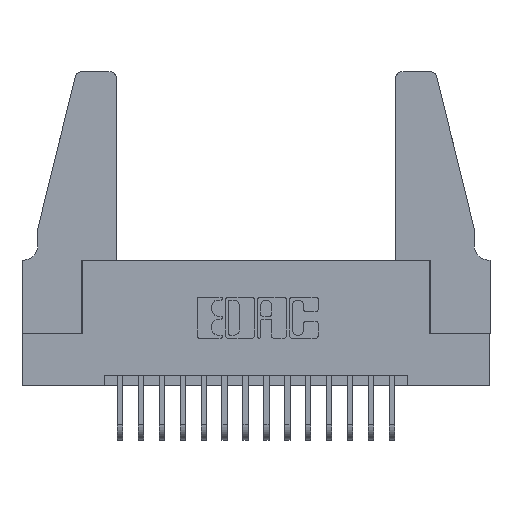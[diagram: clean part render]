
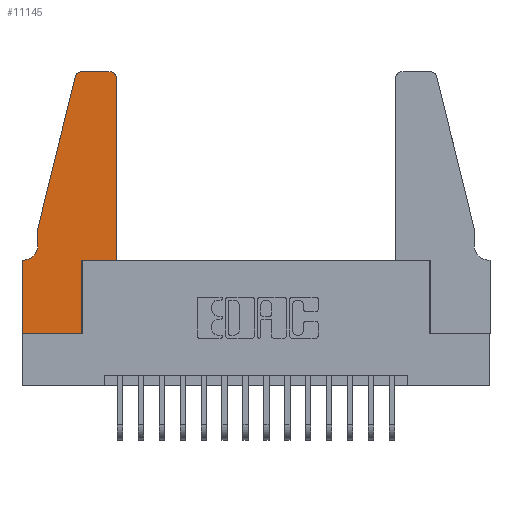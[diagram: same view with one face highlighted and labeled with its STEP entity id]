
A CAD part, top view. The second image highlights one B-rep face of the part: STEP entity #11145.
In plain terms, the highlighted planar face has unit normal (0, 0, 1).
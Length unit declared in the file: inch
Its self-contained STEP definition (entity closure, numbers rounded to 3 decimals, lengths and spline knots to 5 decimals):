
#33 = CARTESIAN_POINT ( 'NONE',  ( 0.2865, 0.35, 0.37 ) ) ;
#201 = ORIENTED_EDGE ( 'NONE', *, *, #2061, .T. ) ;
#203 = CARTESIAN_POINT ( 'NONE',  ( 0.0755, 0.5, 0.37 ) ) ;
#287 = CARTESIAN_POINT ( 'NONE',  ( 0., 0., 0.37 ) ) ;
#403 = CARTESIAN_POINT ( 'NONE',  ( 0.4205, 1.22, 0.37 ) ) ;
#985 = CARTESIAN_POINT ( 'NONE',  ( 0.4505, 0.35, 0.37 ) ) ;
#1179 = ORIENTED_EDGE ( 'NONE', *, *, #13212, .T. ) ;
#1209 = CARTESIAN_POINT ( 'NONE',  ( 0.284, 1.25, 0.37 ) ) ;
#1275 = ORIENTED_EDGE ( 'NONE', *, *, #9316, .T. ) ;
#1276 = LINE ( 'NONE', #287, #14472 ) ;
#1321 = ORIENTED_EDGE ( 'NONE', *, *, #7157, .T. ) ;
#1359 = CARTESIAN_POINT ( 'NONE',  ( 0.4505, 1.22, 0.37 ) ) ;
#1530 = DIRECTION ( 'NONE',  ( 0., -1., 0. ) ) ;
#1729 = DIRECTION ( 'NONE',  ( 1., 0., 0. ) ) ;
#2061 = EDGE_CURVE ( 'NONE', #11973, #10816, #14438, .T. ) ;
#2216 = VERTEX_POINT ( 'NONE', #14817 ) ;
#2221 = AXIS2_PLACEMENT_3D ( 'NONE', #5401, #7891, #14260 ) ;
#2316 = CARTESIAN_POINT ( 'NONE',  ( 0., 0., 0.37 ) ) ;
#2404 = VECTOR ( 'NONE', #12878, 39.37008 ) ;
#2495 = CIRCLE ( 'NONE', #5008, 0.03 ) ;
#2524 = CARTESIAN_POINT ( 'NONE',  ( 0.0755, 0.5, 0.37 ) ) ;
#2651 = LINE ( 'NONE', #13878, #12477 ) ;
#3098 = CARTESIAN_POINT ( 'NONE',  ( 0.0755, 0.42, 0.37 ) ) ;
#3107 = CARTESIAN_POINT ( 'NONE',  ( 0.284, 1.22, 0.37 ) ) ;
#3110 = LINE ( 'NONE', #12853, #9934 ) ;
#3555 = CARTESIAN_POINT ( 'NONE',  ( 0.2865, 0., 0.37 ) ) ;
#3731 = CARTESIAN_POINT ( 'NONE',  ( 0., 0., 0.37 ) ) ;
#3781 = ORIENTED_EDGE ( 'NONE', *, *, #9706, .T. ) ;
#3836 = DIRECTION ( 'NONE',  ( -1., 0., 0. ) ) ;
#3840 = VERTEX_POINT ( 'NONE', #2316 ) ;
#3897 = DIRECTION ( 'NONE',  ( -0.239, -0.971, 0. ) ) ;
#4207 = VECTOR ( 'NONE', #1530, 39.37008 ) ;
#4350 = DIRECTION ( 'NONE',  ( 0., 0., -1. ) ) ;
#4402 = DIRECTION ( 'NONE',  ( 1., 0., 0. ) ) ;
#4858 = VECTOR ( 'NONE', #10003, 39.37008 ) ;
#4940 = VECTOR ( 'NONE', #5510, 39.37008 ) ;
#5008 = AXIS2_PLACEMENT_3D ( 'NONE', #3107, #12085, #4402 ) ;
#5057 = VERTEX_POINT ( 'NONE', #12518 ) ;
#5401 = CARTESIAN_POINT ( 'NONE',  ( 0., 0.35, 0.37 ) ) ;
#5450 = EDGE_CURVE ( 'NONE', #14455, #2216, #13625, .T. ) ;
#5510 = DIRECTION ( 'NONE',  ( -1., 0., 0. ) ) ;
#5614 = VERTEX_POINT ( 'NONE', #3555 ) ;
#5623 = EDGE_CURVE ( 'NONE', #16062, #14455, #7446, .T. ) ;
#5739 = DIRECTION ( 'NONE',  ( -1., 0., 0. ) ) ;
#5833 = FACE_OUTER_BOUND ( 'NONE', #7696, .T. ) ;
#5992 = ORIENTED_EDGE ( 'NONE', *, *, #11619, .T. ) ;
#6297 = DIRECTION ( 'NONE',  ( 1., 0., 0. ) ) ;
#6413 = ORIENTED_EDGE ( 'NONE', *, *, #5450, .T. ) ;
#6820 = LINE ( 'NONE', #3731, #12411 ) ;
#7157 = EDGE_CURVE ( 'NONE', #5614, #10305, #15539, .T. ) ;
#7244 = EDGE_CURVE ( 'NONE', #8904, #11973, #14351, .T. ) ;
#7446 = LINE ( 'NONE', #985, #4858 ) ;
#7658 = ORIENTED_EDGE ( 'NONE', *, *, #9943, .T. ) ;
#7696 = EDGE_LOOP ( 'NONE', ( #1275, #7658, #3781, #8396, #201, #1179, #15959, #5992, #1321, #16173, #15034, #6413 ) ) ;
#7891 = DIRECTION ( 'NONE',  ( 0., 0., 1. ) ) ;
#8396 = ORIENTED_EDGE ( 'NONE', *, *, #7244, .T. ) ;
#8460 = CARTESIAN_POINT ( 'NONE',  ( 0.0055, 0.42, 0.37 ) ) ;
#8904 = VERTEX_POINT ( 'NONE', #2524 ) ;
#9130 = PLANE ( 'NONE',  #2221 ) ;
#9316 = EDGE_CURVE ( 'NONE', #2216, #16002, #11761, .T. ) ;
#9446 = DIRECTION ( 'NONE',  ( 0., 0., 1. ) ) ;
#9706 = EDGE_CURVE ( 'NONE', #12492, #8904, #3110, .T. ) ;
#9781 = AXIS2_PLACEMENT_3D ( 'NONE', #403, #9446, #1729 ) ;
#9934 = VECTOR ( 'NONE', #3897, 39.37008 ) ;
#9943 = EDGE_CURVE ( 'NONE', #16002, #12492, #2495, .T. ) ;
#10003 = DIRECTION ( 'NONE',  ( 0., 1., 0. ) ) ;
#10305 = VERTEX_POINT ( 'NONE', #11402 ) ;
#10816 = VERTEX_POINT ( 'NONE', #13673 ) ;
#10949 = LINE ( 'NONE', #12791, #14284 ) ;
#11145 = ADVANCED_FACE ( 'NONE', ( #5833 ), #9130, .T. ) ;
#11402 = CARTESIAN_POINT ( 'NONE',  ( 0.2865, 0.35, 0.37 ) ) ;
#11440 = CARTESIAN_POINT ( 'NONE',  ( 0.25487, 1.22718, 0.37 ) ) ;
#11619 = EDGE_CURVE ( 'NONE', #3840, #5614, #6820, .T. ) ;
#11761 = LINE ( 'NONE', #15573, #4940 ) ;
#11973 = VERTEX_POINT ( 'NONE', #3098 ) ;
#12085 = DIRECTION ( 'NONE',  ( 0., 0., 1. ) ) ;
#12411 = VECTOR ( 'NONE', #15128, 39.37008 ) ;
#12477 = VECTOR ( 'NONE', #6297, 39.37008 ) ;
#12492 = VERTEX_POINT ( 'NONE', #11440 ) ;
#12518 = CARTESIAN_POINT ( 'NONE',  ( 0., 0.35, 0.37 ) ) ;
#12791 = CARTESIAN_POINT ( 'NONE',  ( 0.0755, 0.35, 0.37 ) ) ;
#12853 = CARTESIAN_POINT ( 'NONE',  ( 0.0755, 0.5, 0.37 ) ) ;
#12878 = DIRECTION ( 'NONE',  ( 0., 1., 0. ) ) ;
#13158 = DIRECTION ( 'NONE',  ( 0., -1., 0. ) ) ;
#13212 = EDGE_CURVE ( 'NONE', #10816, #5057, #10949, .T. ) ;
#13403 = EDGE_CURVE ( 'NONE', #5057, #3840, #1276, .T. ) ;
#13625 = CIRCLE ( 'NONE', #9781, 0.03 ) ;
#13673 = CARTESIAN_POINT ( 'NONE',  ( 0.0055, 0.35, 0.37 ) ) ;
#13878 = CARTESIAN_POINT ( 'NONE',  ( 0.4505, 0.35, 0.37 ) ) ;
#14077 = AXIS2_PLACEMENT_3D ( 'NONE', #8460, #4350, #5739 ) ;
#14124 = CARTESIAN_POINT ( 'NONE',  ( 0.4505, 0.35, 0.37 ) ) ;
#14260 = DIRECTION ( 'NONE',  ( 1., 0., 0. ) ) ;
#14284 = VECTOR ( 'NONE', #3836, 39.37008 ) ;
#14351 = LINE ( 'NONE', #203, #4207 ) ;
#14438 = CIRCLE ( 'NONE', #14077, 0.07 ) ;
#14455 = VERTEX_POINT ( 'NONE', #1359 ) ;
#14472 = VECTOR ( 'NONE', #13158, 39.37008 ) ;
#14817 = CARTESIAN_POINT ( 'NONE',  ( 0.4205, 1.25, 0.37 ) ) ;
#15034 = ORIENTED_EDGE ( 'NONE', *, *, #5623, .T. ) ;
#15128 = DIRECTION ( 'NONE',  ( 1., 0., 0. ) ) ;
#15278 = EDGE_CURVE ( 'NONE', #10305, #16062, #2651, .T. ) ;
#15539 = LINE ( 'NONE', #33, #2404 ) ;
#15573 = CARTESIAN_POINT ( 'NONE',  ( 0.2605, 1.25, 0.37 ) ) ;
#15959 = ORIENTED_EDGE ( 'NONE', *, *, #13403, .T. ) ;
#16002 = VERTEX_POINT ( 'NONE', #1209 ) ;
#16062 = VERTEX_POINT ( 'NONE', #14124 ) ;
#16173 = ORIENTED_EDGE ( 'NONE', *, *, #15278, .T. ) ;
